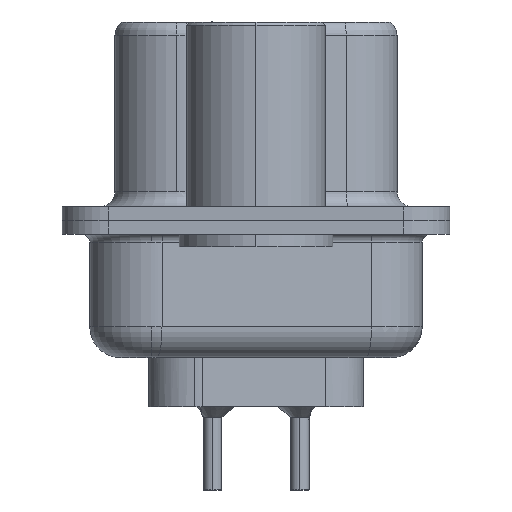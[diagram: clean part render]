
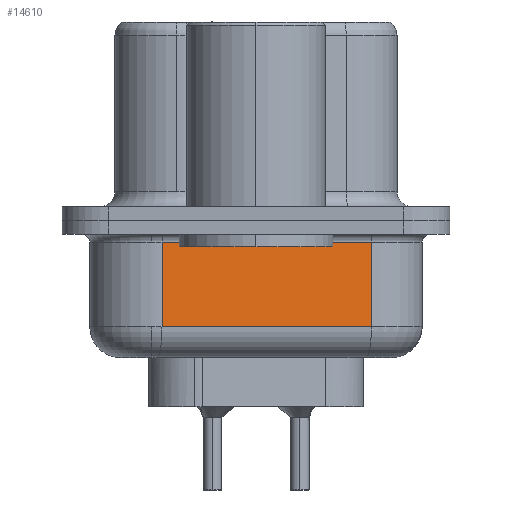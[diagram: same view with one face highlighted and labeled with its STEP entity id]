
A CAD part, left-side view. The second image highlights one B-rep face of the part: STEP entity #14610.
In plain terms, the highlighted planar face has unit normal (-0.985, -0.174, 0).
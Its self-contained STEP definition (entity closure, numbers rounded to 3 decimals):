
#593 = CARTESIAN_POINT ( 'NONE',  ( 2.89, 3.053, -3.45 ) ) ;
#874 = VECTOR ( 'NONE', #7688, 1000. ) ;
#1355 = DIRECTION ( 'NONE',  ( 0., 0., 1. ) ) ;
#4234 = VECTOR ( 'NONE', #8286, 1000. ) ;
#4482 = DIRECTION ( 'NONE',  ( 0.985, 0.174, 0. ) ) ;
#4773 = CARTESIAN_POINT ( 'NONE',  ( 4.089, -3.747, -4.45 ) ) ;
#5458 = LINE ( 'NONE', #17906, #874 ) ;
#6154 = VECTOR ( 'NONE', #1355, 1000. ) ;
#6548 = ORIENTED_EDGE ( 'NONE', *, *, #17506, .T. ) ;
#7515 = CARTESIAN_POINT ( 'NONE',  ( 4.089, -3.747, -3.45 ) ) ;
#7688 = DIRECTION ( 'NONE',  ( -0.174, 0.985, 0. ) ) ;
#7937 = VECTOR ( 'NONE', #14993, 1000. ) ;
#8286 = DIRECTION ( 'NONE',  ( 0.174, -0.985, 0. ) ) ;
#8799 = LINE ( 'NONE', #16793, #4234 ) ;
#9622 = LINE ( 'NONE', #11597, #6154 ) ;
#11271 = PLANE ( 'NONE',  #18549 ) ;
#11597 = CARTESIAN_POINT ( 'NONE',  ( 2.89, 3.053, -4.45 ) ) ;
#11930 = CARTESIAN_POINT ( 'NONE',  ( 4.089, -3.747, -0.7 ) ) ;
#12066 = VERTEX_POINT ( 'NONE', #20382 ) ;
#12347 = VERTEX_POINT ( 'NONE', #593 ) ;
#12456 = LINE ( 'NONE', #4773, #7937 ) ;
#12803 = EDGE_CURVE ( 'NONE', #20880, #12066, #5458, .T. ) ;
#13967 = ORIENTED_EDGE ( 'NONE', *, *, #15766, .F. ) ;
#14610 = ADVANCED_FACE ( 'NONE', ( #19815 ), #11271, .F. ) ;
#14993 = DIRECTION ( 'NONE',  ( 0., 0., 1. ) ) ;
#15034 = VERTEX_POINT ( 'NONE', #7515 ) ;
#15766 = EDGE_CURVE ( 'NONE', #12347, #12066, #9622, .T. ) ;
#16418 = DIRECTION ( 'NONE',  ( -0.174, 0.985, 0. ) ) ;
#16793 = CARTESIAN_POINT ( 'NONE',  ( 2.89, 3.053, -3.45 ) ) ;
#17506 = EDGE_CURVE ( 'NONE', #12347, #15034, #8799, .T. ) ;
#17906 = CARTESIAN_POINT ( 'NONE',  ( 2.89, 3.053, -0.7 ) ) ;
#18059 = CARTESIAN_POINT ( 'NONE',  ( 2.89, 3.053, -4.45 ) ) ;
#18329 = EDGE_LOOP ( 'NONE', ( #13967, #6548, #19705, #21796 ) ) ;
#18549 = AXIS2_PLACEMENT_3D ( 'NONE', #18059, #4482, #16418 ) ;
#19294 = EDGE_CURVE ( 'NONE', #15034, #20880, #12456, .T. ) ;
#19705 = ORIENTED_EDGE ( 'NONE', *, *, #19294, .T. ) ;
#19815 = FACE_OUTER_BOUND ( 'NONE', #18329, .T. ) ;
#20382 = CARTESIAN_POINT ( 'NONE',  ( 2.89, 3.053, -0.7 ) ) ;
#20880 = VERTEX_POINT ( 'NONE', #11930 ) ;
#21796 = ORIENTED_EDGE ( 'NONE', *, *, #12803, .T. ) ;
